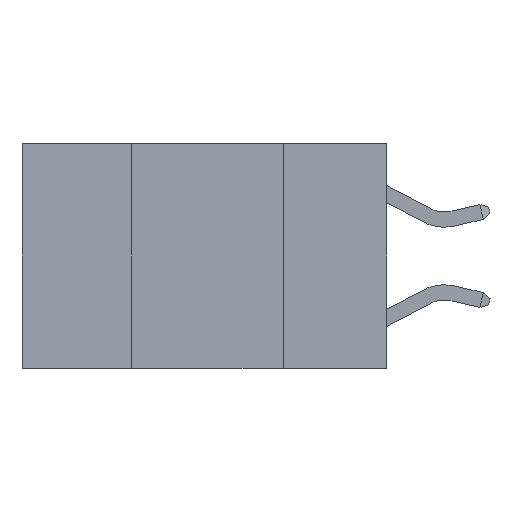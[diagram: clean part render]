
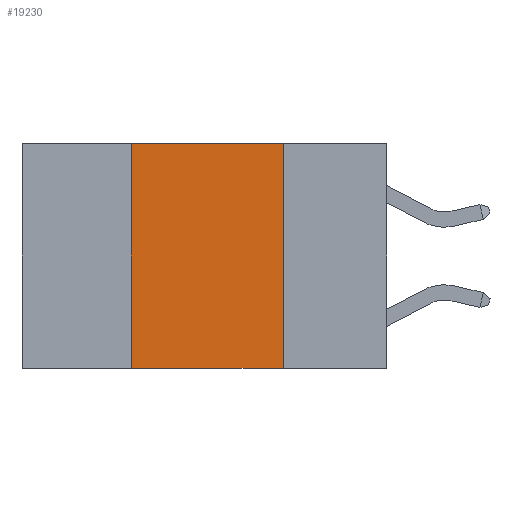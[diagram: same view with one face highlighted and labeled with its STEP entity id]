
A CAD part, left-side view. The second image highlights one B-rep face of the part: STEP entity #19230.
In plain terms, the highlighted planar face has unit normal (-1, 0, 0).
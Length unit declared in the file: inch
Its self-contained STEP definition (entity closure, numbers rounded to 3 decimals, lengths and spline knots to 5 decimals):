
#3744 = VERTEX_POINT ( 'NONE', #19813 ) ;
#3746 = CARTESIAN_POINT ( 'NONE',  ( 0., 0.42, -0.37 ) ) ;
#4674 = CARTESIAN_POINT ( 'NONE',  ( 0., 0.17, 0. ) ) ;
#4679 = VECTOR ( 'NONE', #25336, 39.37008 ) ;
#5413 = VERTEX_POINT ( 'NONE', #21379 ) ;
#5755 = EDGE_CURVE ( 'NONE', #27262, #5413, #24765, .T. ) ;
#8214 = CARTESIAN_POINT ( 'NONE',  ( 0., 0.6, 0. ) ) ;
#8877 = ORIENTED_EDGE ( 'NONE', *, *, #15021, .F. ) ;
#9048 = VERTEX_POINT ( 'NONE', #10215 ) ;
#9309 = DIRECTION ( 'NONE',  ( 0., -1., 0. ) ) ;
#10215 = CARTESIAN_POINT ( 'NONE',  ( 0., 0.17, 0. ) ) ;
#10771 = DIRECTION ( 'NONE',  ( 0., 0., -1. ) ) ;
#10969 = ORIENTED_EDGE ( 'NONE', *, *, #5755, .F. ) ;
#11994 = EDGE_LOOP ( 'NONE', ( #8877, #16051, #10969, #12579 ) ) ;
#12579 = ORIENTED_EDGE ( 'NONE', *, *, #17930, .T. ) ;
#13433 = LINE ( 'NONE', #14717, #26046 ) ;
#14717 = CARTESIAN_POINT ( 'NONE',  ( 0., 0.6, 0. ) ) ;
#15021 = EDGE_CURVE ( 'NONE', #9048, #3744, #20834, .T. ) ;
#16051 = ORIENTED_EDGE ( 'NONE', *, *, #18034, .F. ) ;
#17240 = DIRECTION ( 'NONE',  ( 0., -1., 0. ) ) ;
#17930 = EDGE_CURVE ( 'NONE', #27262, #3744, #30796, .T. ) ;
#18034 = EDGE_CURVE ( 'NONE', #5413, #9048, #13433, .T. ) ;
#19230 = ADVANCED_FACE ( 'NONE', ( #24802 ), #20772, .F. ) ;
#19723 = DIRECTION ( 'NONE',  ( 0., 0., -1. ) ) ;
#19747 = AXIS2_PLACEMENT_3D ( 'NONE', #8214, #25845, #10771 ) ;
#19813 = CARTESIAN_POINT ( 'NONE',  ( 0., 0.17, -0.37 ) ) ;
#20250 = CARTESIAN_POINT ( 'NONE',  ( 0., 0.42, 0. ) ) ;
#20772 = PLANE ( 'NONE',  #19747 ) ;
#20834 = LINE ( 'NONE', #4674, #27551 ) ;
#21379 = CARTESIAN_POINT ( 'NONE',  ( 0., 0.42, 0. ) ) ;
#22515 = VECTOR ( 'NONE', #9309, 39.37008 ) ;
#24765 = LINE ( 'NONE', #20250, #4679 ) ;
#24802 = FACE_OUTER_BOUND ( 'NONE', #11994, .T. ) ;
#25336 = DIRECTION ( 'NONE',  ( 0., 0., 1. ) ) ;
#25845 = DIRECTION ( 'NONE',  ( 1., 0., 0. ) ) ;
#26046 = VECTOR ( 'NONE', #17240, 39.37008 ) ;
#27262 = VERTEX_POINT ( 'NONE', #3746 ) ;
#27551 = VECTOR ( 'NONE', #19723, 39.37008 ) ;
#30796 = LINE ( 'NONE', #31891, #22515 ) ;
#31891 = CARTESIAN_POINT ( 'NONE',  ( 0., 0.6, -0.37 ) ) ;
